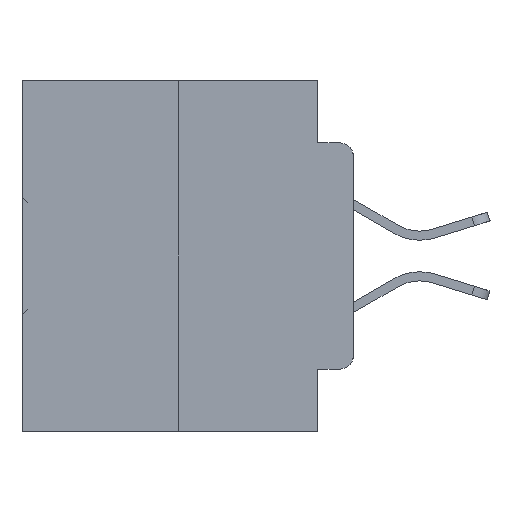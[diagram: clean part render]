
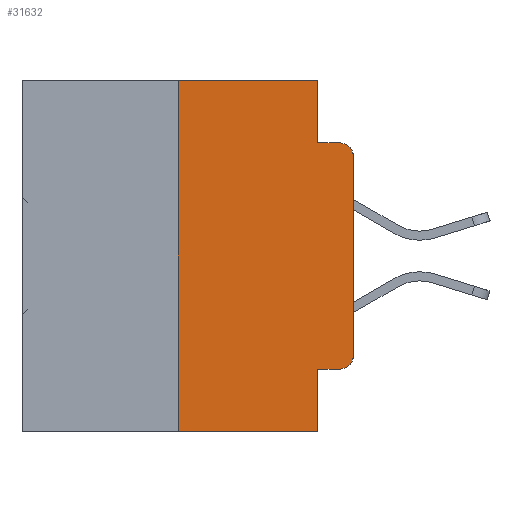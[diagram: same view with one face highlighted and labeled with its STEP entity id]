
A CAD part, left-side view. The second image highlights one B-rep face of the part: STEP entity #31632.
In plain terms, the highlighted planar face has unit normal (-1, 0, 0).
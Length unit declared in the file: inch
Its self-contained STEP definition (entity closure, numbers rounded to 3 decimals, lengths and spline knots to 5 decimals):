
#235 = ORIENTED_EDGE ( 'NONE', *, *, #26155, .F. ) ;
#379 = VERTEX_POINT ( 'NONE', #27535 ) ;
#491 = DIRECTION ( 'NONE',  ( 0., -1., 0. ) ) ;
#1045 = VECTOR ( 'NONE', #2430, 39.37008 ) ;
#1046 = VERTEX_POINT ( 'NONE', #20847 ) ;
#1494 = CARTESIAN_POINT ( 'NONE',  ( 0., 0.02, -0.4115 ) ) ;
#1528 = ORIENTED_EDGE ( 'NONE', *, *, #33386, .F. ) ;
#1815 = EDGE_CURVE ( 'NONE', #17251, #24354, #7576, .T. ) ;
#1911 = DIRECTION ( 'NONE',  ( 1., 0., 0. ) ) ;
#1929 = VERTEX_POINT ( 'NONE', #1494 ) ;
#2430 = DIRECTION ( 'NONE',  ( 0., -1., 0. ) ) ;
#2564 = VECTOR ( 'NONE', #13316, 39.37008 ) ;
#2819 = ORIENTED_EDGE ( 'NONE', *, *, #32696, .T. ) ;
#3821 = VERTEX_POINT ( 'NONE', #34929 ) ;
#4359 = EDGE_CURVE ( 'NONE', #1929, #3821, #33547, .T. ) ;
#4595 = DIRECTION ( 'NONE',  ( 0., -1., 0. ) ) ;
#4956 = VECTOR ( 'NONE', #14474, 39.37008 ) ;
#5066 = DIRECTION ( 'NONE',  ( -1., 0., 0. ) ) ;
#5274 = FACE_OUTER_BOUND ( 'NONE', #34638, .T. ) ;
#5769 = CARTESIAN_POINT ( 'NONE',  ( 0., 0.02, -0.3915 ) ) ;
#6003 = VECTOR ( 'NONE', #19827, 39.37008 ) ;
#6277 = ORIENTED_EDGE ( 'NONE', *, *, #13478, .T. ) ;
#6975 = DIRECTION ( 'NONE',  ( 0., 0., -1. ) ) ;
#7058 = DIRECTION ( 'NONE',  ( -1., 0., 0. ) ) ;
#7576 = LINE ( 'NONE', #14260, #21164 ) ;
#7612 = VECTOR ( 'NONE', #12789, 39.37008 ) ;
#7977 = ORIENTED_EDGE ( 'NONE', *, *, #4359, .T. ) ;
#8186 = LINE ( 'NONE', #34706, #14553 ) ;
#9300 = VERTEX_POINT ( 'NONE', #18124 ) ;
#9715 = CARTESIAN_POINT ( 'NONE',  ( 0., 0.25, -0.5 ) ) ;
#9945 = CARTESIAN_POINT ( 'NONE',  ( 0., 0.473, 0. ) ) ;
#10286 = EDGE_CURVE ( 'NONE', #3821, #20563, #21300, .T. ) ;
#12186 = LINE ( 'NONE', #17090, #4956 ) ;
#12789 = DIRECTION ( 'NONE',  ( 0., 0., 1. ) ) ;
#13099 = EDGE_CURVE ( 'NONE', #24253, #9300, #12186, .T. ) ;
#13316 = DIRECTION ( 'NONE',  ( 0., 0., -1. ) ) ;
#13362 = EDGE_CURVE ( 'NONE', #1046, #30734, #13463, .T. ) ;
#13463 = LINE ( 'NONE', #9945, #18121 ) ;
#13478 = EDGE_CURVE ( 'NONE', #379, #1929, #22751, .T. ) ;
#14260 = CARTESIAN_POINT ( 'NONE',  ( 0., 0.051, -0.0885 ) ) ;
#14319 = ORIENTED_EDGE ( 'NONE', *, *, #1815, .F. ) ;
#14474 = DIRECTION ( 'NONE',  ( 0., -1., 0. ) ) ;
#14553 = VECTOR ( 'NONE', #21276, 39.37008 ) ;
#14657 = AXIS2_PLACEMENT_3D ( 'NONE', #21314, #5066, #24019 ) ;
#17090 = CARTESIAN_POINT ( 'NONE',  ( 0., 0.473, -0.5 ) ) ;
#17114 = CARTESIAN_POINT ( 'NONE',  ( 0., 0., 0. ) ) ;
#17251 = VERTEX_POINT ( 'NONE', #32562 ) ;
#17710 = ORIENTED_EDGE ( 'NONE', *, *, #10286, .T. ) ;
#18121 = VECTOR ( 'NONE', #4595, 39.37008 ) ;
#18124 = CARTESIAN_POINT ( 'NONE',  ( 0., 0.051, -0.5 ) ) ;
#18168 = ORIENTED_EDGE ( 'NONE', *, *, #20747, .F. ) ;
#18221 = PLANE ( 'NONE',  #31817 ) ;
#19827 = DIRECTION ( 'NONE',  ( 0., 0., 1. ) ) ;
#20563 = VERTEX_POINT ( 'NONE', #25973 ) ;
#20747 = EDGE_CURVE ( 'NONE', #379, #9300, #31378, .T. ) ;
#20847 = CARTESIAN_POINT ( 'NONE',  ( 0., 0.25, 0. ) ) ;
#20953 = DIRECTION ( 'NONE',  ( 0., 0., -1. ) ) ;
#21164 = VECTOR ( 'NONE', #491, 39.37008 ) ;
#21276 = DIRECTION ( 'NONE',  ( 0., 0., -1. ) ) ;
#21300 = LINE ( 'NONE', #17114, #6003 ) ;
#21314 = CARTESIAN_POINT ( 'NONE',  ( 0., 0.02, -0.1085 ) ) ;
#21439 = CARTESIAN_POINT ( 'NONE',  ( 0., 0.051, -0.4115 ) ) ;
#22751 = LINE ( 'NONE', #21439, #1045 ) ;
#23652 = ORIENTED_EDGE ( 'NONE', *, *, #13099, .T. ) ;
#24019 = DIRECTION ( 'NONE',  ( 0., 0., -1. ) ) ;
#24253 = VERTEX_POINT ( 'NONE', #9715 ) ;
#24354 = VERTEX_POINT ( 'NONE', #34289 ) ;
#25379 = AXIS2_PLACEMENT_3D ( 'NONE', #5769, #7058, #6975 ) ;
#25973 = CARTESIAN_POINT ( 'NONE',  ( 0., 0., -0.1085 ) ) ;
#26155 = EDGE_CURVE ( 'NONE', #24253, #1046, #34687, .T. ) ;
#26269 = CARTESIAN_POINT ( 'NONE',  ( 0., 0.25, 0. ) ) ;
#27535 = CARTESIAN_POINT ( 'NONE',  ( 0., 0.051, -0.4115 ) ) ;
#27968 = CARTESIAN_POINT ( 'NONE',  ( 0., 0.051, 0. ) ) ;
#28934 = CIRCLE ( 'NONE', #14657, 0.02 ) ;
#30734 = VERTEX_POINT ( 'NONE', #27968 ) ;
#31217 = ORIENTED_EDGE ( 'NONE', *, *, #13362, .F. ) ;
#31378 = LINE ( 'NONE', #31976, #2564 ) ;
#31632 = ADVANCED_FACE ( 'NONE', ( #5274 ), #18221, .F. ) ;
#31657 = CARTESIAN_POINT ( 'NONE',  ( 0., 0.473, 0. ) ) ;
#31817 = AXIS2_PLACEMENT_3D ( 'NONE', #31657, #1911, #20953 ) ;
#31976 = CARTESIAN_POINT ( 'NONE',  ( 0., 0.051, 0. ) ) ;
#32562 = CARTESIAN_POINT ( 'NONE',  ( 0., 0.051, -0.0885 ) ) ;
#32696 = EDGE_CURVE ( 'NONE', #20563, #24354, #28934, .T. ) ;
#33386 = EDGE_CURVE ( 'NONE', #30734, #17251, #8186, .T. ) ;
#33547 = CIRCLE ( 'NONE', #25379, 0.02 ) ;
#34289 = CARTESIAN_POINT ( 'NONE',  ( 0., 0.02, -0.0885 ) ) ;
#34638 = EDGE_LOOP ( 'NONE', ( #17710, #2819, #14319, #1528, #31217, #235, #23652, #18168, #6277, #7977 ) ) ;
#34687 = LINE ( 'NONE', #26269, #7612 ) ;
#34706 = CARTESIAN_POINT ( 'NONE',  ( 0., 0.051, 0. ) ) ;
#34929 = CARTESIAN_POINT ( 'NONE',  ( 0., 0., -0.3915 ) ) ;
